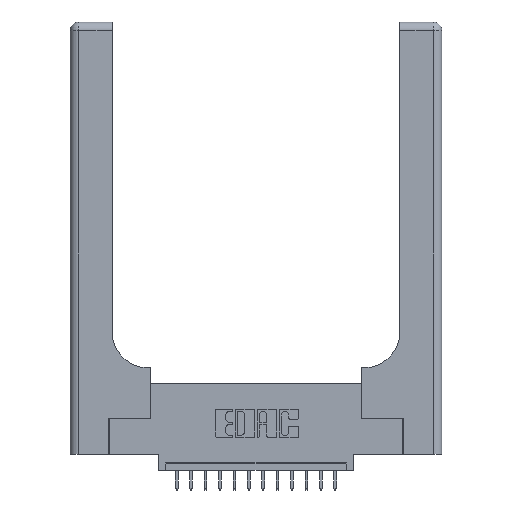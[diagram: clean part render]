
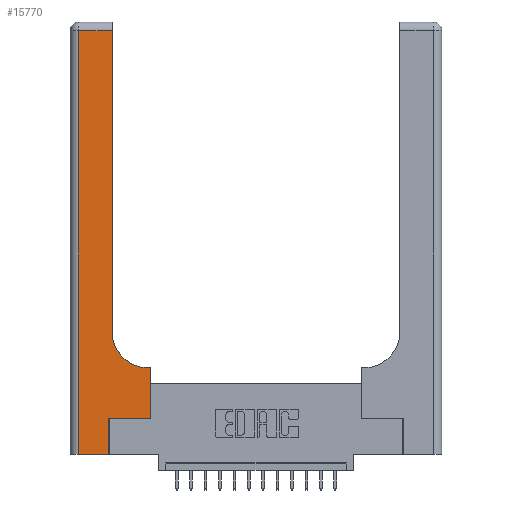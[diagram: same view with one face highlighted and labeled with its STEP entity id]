
A CAD part, top view. The second image highlights one B-rep face of the part: STEP entity #15770.
In plain terms, the highlighted planar face has unit normal (0, 0, 1).
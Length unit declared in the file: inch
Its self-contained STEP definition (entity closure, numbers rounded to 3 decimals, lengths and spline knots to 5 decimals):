
#106 = EDGE_CURVE ( 'NONE', #12677, #4206, #5439, .T. ) ;
#179 = VERTEX_POINT ( 'NONE', #7146 ) ;
#285 = ORIENTED_EDGE ( 'NONE', *, *, #14459, .T. ) ;
#500 = ORIENTED_EDGE ( 'NONE', *, *, #4194, .T. ) ;
#1017 = CARTESIAN_POINT ( 'NONE',  ( 0.2915, 3., 0.37 ) ) ;
#1113 = EDGE_LOOP ( 'NONE', ( #15774, #12735, #3203, #11475, #13946, #285, #9237, #500, #12506 ) ) ;
#1750 = VECTOR ( 'NONE', #2509, 39.37008 ) ;
#2019 = EDGE_CURVE ( 'NONE', #15474, #179, #5257, .T. ) ;
#2120 = VECTOR ( 'NONE', #17753, 39.37008 ) ;
#2509 = DIRECTION ( 'NONE',  ( -1., 0., 0. ) ) ;
#3179 = LINE ( 'NONE', #14761, #2120 ) ;
#3203 = ORIENTED_EDGE ( 'NONE', *, *, #6951, .T. ) ;
#4194 = EDGE_CURVE ( 'NONE', #7114, #15474, #7948, .T. ) ;
#4206 = VERTEX_POINT ( 'NONE', #12994 ) ;
#5257 = CIRCLE ( 'NONE', #5543, 0.25 ) ;
#5282 = DIRECTION ( 'NONE',  ( 0., 1., 0. ) ) ;
#5286 = VERTEX_POINT ( 'NONE', #7068 ) ;
#5294 = CARTESIAN_POINT ( 'NONE',  ( 0.5415, 0.85, 0.37 ) ) ;
#5346 = CARTESIAN_POINT ( 'NONE',  ( 0.269, 0., 0.37 ) ) ;
#5439 = LINE ( 'NONE', #5346, #15414 ) ;
#5543 = AXIS2_PLACEMENT_3D ( 'NONE', #5294, #12426, #16717 ) ;
#5764 = CARTESIAN_POINT ( 'NONE',  ( 0.5415, 0.6, 0.37 ) ) ;
#6325 = VECTOR ( 'NONE', #12387, 39.37008 ) ;
#6384 = CARTESIAN_POINT ( 'NONE',  ( 0.269, 0.25, 0.37 ) ) ;
#6476 = CARTESIAN_POINT ( 'NONE',  ( 0.5585, 0.25, 0.37 ) ) ;
#6532 = DIRECTION ( 'NONE',  ( 0., -1., 0. ) ) ;
#6772 = EDGE_CURVE ( 'NONE', #7004, #12677, #3179, .T. ) ;
#6951 = EDGE_CURVE ( 'NONE', #5286, #7004, #10733, .T. ) ;
#7004 = VERTEX_POINT ( 'NONE', #14121 ) ;
#7068 = CARTESIAN_POINT ( 'NONE',  ( 0.06, 2.94, 0.37 ) ) ;
#7114 = VERTEX_POINT ( 'NONE', #14212 ) ;
#7146 = CARTESIAN_POINT ( 'NONE',  ( 0.2915, 0.85, 0.37 ) ) ;
#7948 = LINE ( 'NONE', #12429, #1750 ) ;
#8161 = CARTESIAN_POINT ( 'NONE',  ( 0.06, 3., 0.37 ) ) ;
#8176 = CARTESIAN_POINT ( 'NONE',  ( 0.2915, 2.94, 0.37 ) ) ;
#8662 = DIRECTION ( 'NONE',  ( -1., 0., 0. ) ) ;
#9237 = ORIENTED_EDGE ( 'NONE', *, *, #10176, .T. ) ;
#9284 = VECTOR ( 'NONE', #6532, 39.37008 ) ;
#9355 = LINE ( 'NONE', #12536, #10485 ) ;
#9538 = EDGE_CURVE ( 'NONE', #14881, #5286, #9355, .T. ) ;
#9586 = LINE ( 'NONE', #6476, #6325 ) ;
#10176 = EDGE_CURVE ( 'NONE', #12045, #7114, #9586, .T. ) ;
#10485 = VECTOR ( 'NONE', #16537, 39.37008 ) ;
#10733 = LINE ( 'NONE', #8161, #9284 ) ;
#11064 = DIRECTION ( 'NONE',  ( 0., 1., 0. ) ) ;
#11475 = ORIENTED_EDGE ( 'NONE', *, *, #6772, .T. ) ;
#11958 = CARTESIAN_POINT ( 'NONE',  ( 0.5585, 0.25, 0.37 ) ) ;
#12045 = VERTEX_POINT ( 'NONE', #11958 ) ;
#12180 = LINE ( 'NONE', #6384, #13375 ) ;
#12387 = DIRECTION ( 'NONE',  ( 0., 1., 0. ) ) ;
#12426 = DIRECTION ( 'NONE',  ( 0., 0., -1. ) ) ;
#12429 = CARTESIAN_POINT ( 'NONE',  ( 0.2915, 0.6, 0.37 ) ) ;
#12506 = ORIENTED_EDGE ( 'NONE', *, *, #2019, .T. ) ;
#12523 = AXIS2_PLACEMENT_3D ( 'NONE', #15664, #12961, #8662 ) ;
#12536 = CARTESIAN_POINT ( 'NONE',  ( 0., 2.94, 0.37 ) ) ;
#12677 = VERTEX_POINT ( 'NONE', #17861 ) ;
#12735 = ORIENTED_EDGE ( 'NONE', *, *, #9538, .T. ) ;
#12961 = DIRECTION ( 'NONE',  ( 0., 0., -1. ) ) ;
#12994 = CARTESIAN_POINT ( 'NONE',  ( 0.269, 0.25, 0.37 ) ) ;
#13375 = VECTOR ( 'NONE', #13798, 39.37008 ) ;
#13517 = EDGE_CURVE ( 'NONE', #179, #14881, #13832, .T. ) ;
#13798 = DIRECTION ( 'NONE',  ( 1., 0., 0. ) ) ;
#13832 = LINE ( 'NONE', #1017, #13904 ) ;
#13904 = VECTOR ( 'NONE', #5282, 39.37008 ) ;
#13946 = ORIENTED_EDGE ( 'NONE', *, *, #106, .T. ) ;
#14121 = CARTESIAN_POINT ( 'NONE',  ( 0.06, 0., 0.37 ) ) ;
#14180 = PLANE ( 'NONE',  #12523 ) ;
#14212 = CARTESIAN_POINT ( 'NONE',  ( 0.5585, 0.6, 0.37 ) ) ;
#14459 = EDGE_CURVE ( 'NONE', #4206, #12045, #12180, .T. ) ;
#14761 = CARTESIAN_POINT ( 'NONE',  ( 0., 0., 0.37 ) ) ;
#14881 = VERTEX_POINT ( 'NONE', #8176 ) ;
#15414 = VECTOR ( 'NONE', #11064, 39.37008 ) ;
#15474 = VERTEX_POINT ( 'NONE', #5764 ) ;
#15664 = CARTESIAN_POINT ( 'NONE',  ( 0., 3., 0.37 ) ) ;
#15770 = ADVANCED_FACE ( 'NONE', ( #17145 ), #14180, .F. ) ;
#15774 = ORIENTED_EDGE ( 'NONE', *, *, #13517, .T. ) ;
#16537 = DIRECTION ( 'NONE',  ( -1., 0., 0. ) ) ;
#16717 = DIRECTION ( 'NONE',  ( 1., 0., 0. ) ) ;
#17145 = FACE_OUTER_BOUND ( 'NONE', #1113, .T. ) ;
#17753 = DIRECTION ( 'NONE',  ( 1., 0., 0. ) ) ;
#17861 = CARTESIAN_POINT ( 'NONE',  ( 0.269, 0., 0.37 ) ) ;
